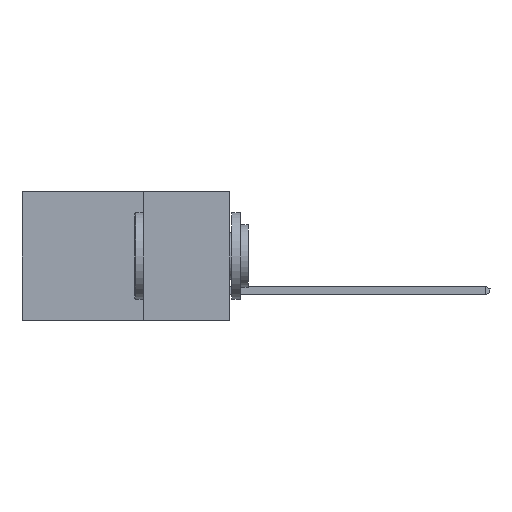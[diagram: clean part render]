
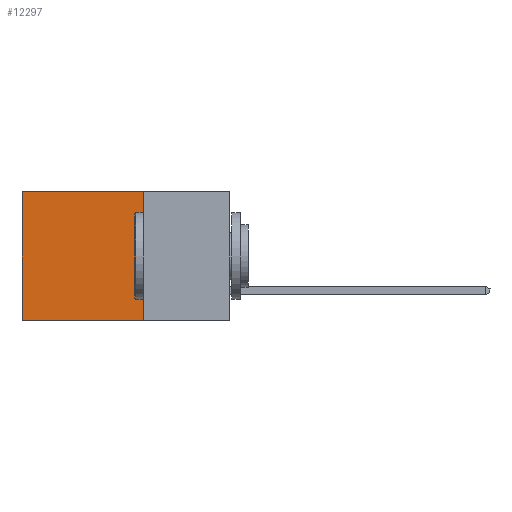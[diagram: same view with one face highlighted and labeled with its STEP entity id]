
A CAD part, left-side view. The second image highlights one B-rep face of the part: STEP entity #12297.
In plain terms, the highlighted planar face has unit normal (-1, 0, 0).
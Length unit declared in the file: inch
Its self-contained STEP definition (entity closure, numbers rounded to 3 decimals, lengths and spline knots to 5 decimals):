
#1015 = LINE ( 'NONE', #18575, #10504 ) ;
#2825 = DIRECTION ( 'NONE',  ( 0., 1., 0. ) ) ;
#3806 = EDGE_CURVE ( 'NONE', #5478, #21667, #19962, .T. ) ;
#3866 = FACE_OUTER_BOUND ( 'NONE', #12688, .T. ) ;
#4456 = ORIENTED_EDGE ( 'NONE', *, *, #21063, .F. ) ;
#5305 = EDGE_CURVE ( 'NONE', #5478, #5729, #21476, .T. ) ;
#5478 = VERTEX_POINT ( 'NONE', #15086 ) ;
#5631 = CARTESIAN_POINT ( 'NONE',  ( 0.2615, 0.25, 0. ) ) ;
#5729 = VERTEX_POINT ( 'NONE', #18462 ) ;
#5754 = DIRECTION ( 'NONE',  ( 0., 1., 0. ) ) ;
#6125 = ORIENTED_EDGE ( 'NONE', *, *, #3806, .F. ) ;
#6893 = VERTEX_POINT ( 'NONE', #11668 ) ;
#7911 = CARTESIAN_POINT ( 'NONE',  ( 0.2615, 0.6, -0.37 ) ) ;
#8083 = EDGE_CURVE ( 'NONE', #5729, #6893, #12922, .T. ) ;
#8454 = AXIS2_PLACEMENT_3D ( 'NONE', #19624, #10935, #17893 ) ;
#10504 = VECTOR ( 'NONE', #2825, 39.37008 ) ;
#10935 = DIRECTION ( 'NONE',  ( 1., 0., 0. ) ) ;
#11668 = CARTESIAN_POINT ( 'NONE',  ( 0.2615, 0.6, -0.37 ) ) ;
#12297 = ADVANCED_FACE ( 'NONE', ( #3866 ), #17786, .F. ) ;
#12688 = EDGE_LOOP ( 'NONE', ( #18278, #4456, #6125, #15123 ) ) ;
#12922 = LINE ( 'NONE', #7911, #21427 ) ;
#13339 = DIRECTION ( 'NONE',  ( 0., 0., -1. ) ) ;
#14871 = DIRECTION ( 'NONE',  ( 0., 0., -1. ) ) ;
#15086 = CARTESIAN_POINT ( 'NONE',  ( 0.2615, 0.25, 0. ) ) ;
#15123 = ORIENTED_EDGE ( 'NONE', *, *, #5305, .T. ) ;
#16242 = VECTOR ( 'NONE', #5754, 39.37008 ) ;
#17786 = PLANE ( 'NONE',  #8454 ) ;
#17893 = DIRECTION ( 'NONE',  ( 0., 0., -1. ) ) ;
#18278 = ORIENTED_EDGE ( 'NONE', *, *, #8083, .T. ) ;
#18462 = CARTESIAN_POINT ( 'NONE',  ( 0.2615, 0.6, 0. ) ) ;
#18575 = CARTESIAN_POINT ( 'NONE',  ( 0.2615, 0.25, -0.37 ) ) ;
#18798 = VECTOR ( 'NONE', #13339, 39.37008 ) ;
#19624 = CARTESIAN_POINT ( 'NONE',  ( 0.2615, 0.25, -0.37 ) ) ;
#19962 = LINE ( 'NONE', #20303, #18798 ) ;
#20303 = CARTESIAN_POINT ( 'NONE',  ( 0.2615, 0.25, -0.37 ) ) ;
#20901 = CARTESIAN_POINT ( 'NONE',  ( 0.2615, 0.25, -0.37 ) ) ;
#21063 = EDGE_CURVE ( 'NONE', #21667, #6893, #1015, .T. ) ;
#21427 = VECTOR ( 'NONE', #14871, 39.37008 ) ;
#21476 = LINE ( 'NONE', #5631, #16242 ) ;
#21667 = VERTEX_POINT ( 'NONE', #20901 ) ;
